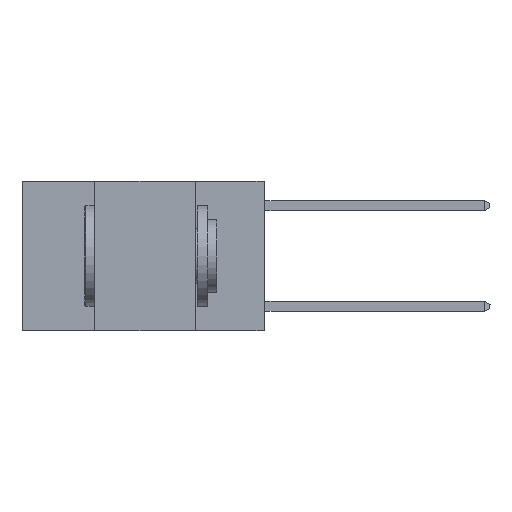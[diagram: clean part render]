
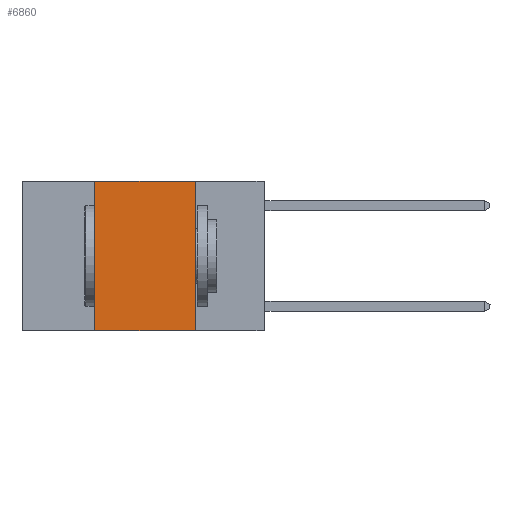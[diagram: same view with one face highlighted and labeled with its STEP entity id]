
A CAD part, left-side view. The second image highlights one B-rep face of the part: STEP entity #6860.
In plain terms, the highlighted planar face has unit normal (-1, 0, 0).
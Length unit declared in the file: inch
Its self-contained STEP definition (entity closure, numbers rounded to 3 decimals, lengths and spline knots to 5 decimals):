
#1209 = LINE ( 'NONE', #6632, #9120 ) ;
#1279 = CARTESIAN_POINT ( 'NONE',  ( 0., 0.17, -0.37 ) ) ;
#1562 = EDGE_CURVE ( 'NONE', #9014, #6741, #5967, .T. ) ;
#1659 = AXIS2_PLACEMENT_3D ( 'NONE', #8851, #10282, #5813 ) ;
#2171 = CARTESIAN_POINT ( 'NONE',  ( 0., 0.17, 0. ) ) ;
#2760 = VECTOR ( 'NONE', #8795, 39.37008 ) ;
#3004 = EDGE_CURVE ( 'NONE', #6741, #8972, #3043, .T. ) ;
#3043 = LINE ( 'NONE', #8864, #2760 ) ;
#3094 = ORIENTED_EDGE ( 'NONE', *, *, #4875, .F. ) ;
#3137 = ORIENTED_EDGE ( 'NONE', *, *, #3004, .F. ) ;
#3240 = ORIENTED_EDGE ( 'NONE', *, *, #1562, .F. ) ;
#3305 = ORIENTED_EDGE ( 'NONE', *, *, #9159, .T. ) ;
#3313 = DIRECTION ( 'NONE',  ( 0., -1., 0. ) ) ;
#4462 = VECTOR ( 'NONE', #7993, 39.37008 ) ;
#4813 = CARTESIAN_POINT ( 'NONE',  ( 0., 0.42, -0.37 ) ) ;
#4875 = EDGE_CURVE ( 'NONE', #8972, #8950, #6648, .T. ) ;
#4988 = PLANE ( 'NONE',  #1659 ) ;
#5346 = DIRECTION ( 'NONE',  ( 0., 0., 1. ) ) ;
#5446 = CARTESIAN_POINT ( 'NONE',  ( 0., 0.42, 0. ) ) ;
#5692 = VECTOR ( 'NONE', #5346, 39.37008 ) ;
#5813 = DIRECTION ( 'NONE',  ( 0., 0., -1. ) ) ;
#5849 = FACE_OUTER_BOUND ( 'NONE', #8905, .T. ) ;
#5967 = LINE ( 'NONE', #5446, #5692 ) ;
#6632 = CARTESIAN_POINT ( 'NONE',  ( 0., 0.6, -0.37 ) ) ;
#6648 = LINE ( 'NONE', #7957, #4462 ) ;
#6741 = VERTEX_POINT ( 'NONE', #7984 ) ;
#6860 = ADVANCED_FACE ( 'NONE', ( #5849 ), #4988, .F. ) ;
#7957 = CARTESIAN_POINT ( 'NONE',  ( 0., 0.17, 0. ) ) ;
#7984 = CARTESIAN_POINT ( 'NONE',  ( 0., 0.42, 0. ) ) ;
#7993 = DIRECTION ( 'NONE',  ( 0., 0., -1. ) ) ;
#8795 = DIRECTION ( 'NONE',  ( 0., -1., 0. ) ) ;
#8851 = CARTESIAN_POINT ( 'NONE',  ( 0., 0.6, 0. ) ) ;
#8864 = CARTESIAN_POINT ( 'NONE',  ( 0., 0.6, 0. ) ) ;
#8905 = EDGE_LOOP ( 'NONE', ( #3094, #3137, #3240, #3305 ) ) ;
#8950 = VERTEX_POINT ( 'NONE', #1279 ) ;
#8972 = VERTEX_POINT ( 'NONE', #2171 ) ;
#9014 = VERTEX_POINT ( 'NONE', #4813 ) ;
#9120 = VECTOR ( 'NONE', #3313, 39.37008 ) ;
#9159 = EDGE_CURVE ( 'NONE', #9014, #8950, #1209, .T. ) ;
#10282 = DIRECTION ( 'NONE',  ( 1., 0., 0. ) ) ;
